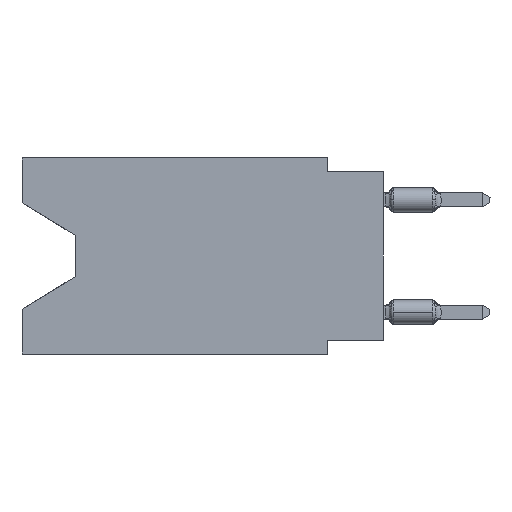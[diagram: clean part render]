
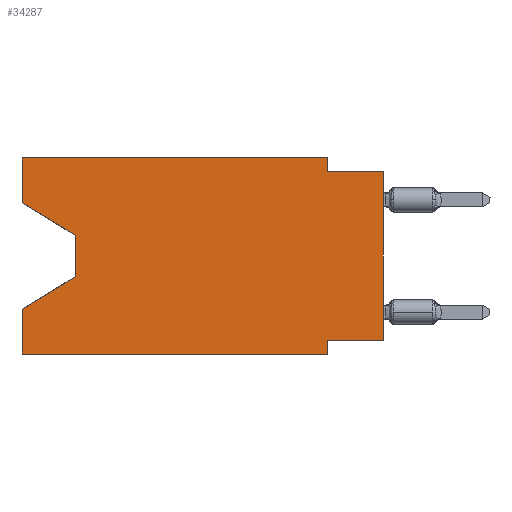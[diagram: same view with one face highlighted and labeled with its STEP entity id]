
A CAD part, left-side view. The second image highlights one B-rep face of the part: STEP entity #34287.
In plain terms, the highlighted planar face has unit normal (-1, 0, 0).
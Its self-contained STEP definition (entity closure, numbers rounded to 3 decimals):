
#469 = ORIENTED_EDGE ( 'NONE', *, *, #32778, .F. ) ;
#590 = FACE_OUTER_BOUND ( 'NONE', #2117, .T. ) ;
#646 = EDGE_CURVE ( 'NONE', #11624, #26078, #7148, .T. ) ;
#716 = ORIENTED_EDGE ( 'NONE', *, *, #38335, .T. ) ;
#778 = VERTEX_POINT ( 'NONE', #39962 ) ;
#858 = ORIENTED_EDGE ( 'NONE', *, *, #14081, .F. ) ;
#910 = CARTESIAN_POINT ( 'NONE',  ( 0., 16.383, 0. ) ) ;
#954 = LINE ( 'NONE', #35859, #6596 ) ;
#1358 = VECTOR ( 'NONE', #21196, 1000. ) ;
#1748 = CARTESIAN_POINT ( 'NONE',  ( 0., 13.97, -5.385 ) ) ;
#1871 = LINE ( 'NONE', #11490, #7334 ) ;
#2117 = EDGE_LOOP ( 'NONE', ( #20671, #716, #14573, #31623, #4939, #858, #12662, #27804, #28840, #469, #36798, #38176 ) ) ;
#2161 = LINE ( 'NONE', #33700, #25986 ) ;
#2420 = LINE ( 'NONE', #15163, #4407 ) ;
#3479 = DIRECTION ( 'NONE',  ( 0., 0., -1. ) ) ;
#3521 = EDGE_CURVE ( 'NONE', #37720, #25284, #1871, .T. ) ;
#4067 = VERTEX_POINT ( 'NONE', #38963 ) ;
#4234 = EDGE_CURVE ( 'NONE', #17017, #778, #39991, .T. ) ;
#4407 = VECTOR ( 'NONE', #27920, 1000. ) ;
#4557 = CARTESIAN_POINT ( 'NONE',  ( 0., 16.383, -8.89 ) ) ;
#4939 = ORIENTED_EDGE ( 'NONE', *, *, #33364, .T. ) ;
#5390 = VECTOR ( 'NONE', #20342, 1000. ) ;
#6102 = CARTESIAN_POINT ( 'NONE',  ( 0., 2.54, 0. ) ) ;
#6384 = VECTOR ( 'NONE', #31040, 1000. ) ;
#6531 = VECTOR ( 'NONE', #20181, 1000. ) ;
#6596 = VECTOR ( 'NONE', #3479, 1000. ) ;
#6736 = DIRECTION ( 'NONE',  ( 0., 0., 1. ) ) ;
#7148 = LINE ( 'NONE', #23651, #18880 ) ;
#7334 = VECTOR ( 'NONE', #12125, 1000. ) ;
#7954 = VECTOR ( 'NONE', #6736, 1000. ) ;
#7988 = CARTESIAN_POINT ( 'NONE',  ( 0., 0., -8.255 ) ) ;
#8026 = CARTESIAN_POINT ( 'NONE',  ( 0., 16.383, 0. ) ) ;
#8684 = CARTESIAN_POINT ( 'NONE',  ( 0., 2.54, 0. ) ) ;
#10314 = CARTESIAN_POINT ( 'NONE',  ( 0., 2.54, -8.255 ) ) ;
#11335 = VERTEX_POINT ( 'NONE', #14252 ) ;
#11345 = EDGE_CURVE ( 'NONE', #4067, #39904, #26813, .T. ) ;
#11490 = CARTESIAN_POINT ( 'NONE',  ( 0., 0., -0.635 ) ) ;
#11589 = CARTESIAN_POINT ( 'NONE',  ( 0., 16.383, 0. ) ) ;
#11623 = LINE ( 'NONE', #30629, #28536 ) ;
#11624 = VERTEX_POINT ( 'NONE', #38499 ) ;
#12125 = DIRECTION ( 'NONE',  ( 0., -1., 0. ) ) ;
#12662 = ORIENTED_EDGE ( 'NONE', *, *, #11345, .F. ) ;
#13435 = DIRECTION ( 'NONE',  ( 0., -0.855, -0.519 ) ) ;
#14081 = EDGE_CURVE ( 'NONE', #39904, #11335, #2161, .T. ) ;
#14186 = EDGE_CURVE ( 'NONE', #4067, #25284, #34133, .T. ) ;
#14252 = CARTESIAN_POINT ( 'NONE',  ( 0., 2.54, -8.89 ) ) ;
#14573 = ORIENTED_EDGE ( 'NONE', *, *, #30015, .T. ) ;
#14727 = LINE ( 'NONE', #11589, #1358 ) ;
#15163 = CARTESIAN_POINT ( 'NONE',  ( 0., 16.383, -8.89 ) ) ;
#17017 = VERTEX_POINT ( 'NONE', #4557 ) ;
#17261 = VERTEX_POINT ( 'NONE', #18448 ) ;
#18448 = CARTESIAN_POINT ( 'NONE',  ( 0., 16.383, 0. ) ) ;
#18880 = VECTOR ( 'NONE', #13435, 1000. ) ;
#19621 = CARTESIAN_POINT ( 'NONE',  ( 0., 16.383, 0. ) ) ;
#20181 = DIRECTION ( 'NONE',  ( 0., 0., 1. ) ) ;
#20342 = DIRECTION ( 'NONE',  ( 0., 0., 1. ) ) ;
#20671 = ORIENTED_EDGE ( 'NONE', *, *, #646, .T. ) ;
#20745 = DIRECTION ( 'NONE',  ( 0., 1., 0. ) ) ;
#21196 = DIRECTION ( 'NONE',  ( 0., -1., 0. ) ) ;
#23651 = CARTESIAN_POINT ( 'NONE',  ( 0., 16.383, -2.038 ) ) ;
#24073 = CARTESIAN_POINT ( 'NONE',  ( 0., 2.54, -0.635 ) ) ;
#24366 = DIRECTION ( 'NONE',  ( 0., 0.855, -0.519 ) ) ;
#25284 = VERTEX_POINT ( 'NONE', #40698 ) ;
#25986 = VECTOR ( 'NONE', #31192, 1000. ) ;
#26078 = VERTEX_POINT ( 'NONE', #29476 ) ;
#26813 = LINE ( 'NONE', #7988, #39894 ) ;
#27233 = CARTESIAN_POINT ( 'NONE',  ( 0., 0., 0. ) ) ;
#27804 = ORIENTED_EDGE ( 'NONE', *, *, #14186, .T. ) ;
#27920 = DIRECTION ( 'NONE',  ( 0., -1., 0. ) ) ;
#28199 = EDGE_CURVE ( 'NONE', #17261, #41174, #14727, .T. ) ;
#28536 = VECTOR ( 'NONE', #24366, 1000. ) ;
#28840 = ORIENTED_EDGE ( 'NONE', *, *, #3521, .F. ) ;
#29476 = CARTESIAN_POINT ( 'NONE',  ( 0., 13.97, -3.505 ) ) ;
#30015 = EDGE_CURVE ( 'NONE', #30370, #778, #11623, .T. ) ;
#30370 = VERTEX_POINT ( 'NONE', #1748 ) ;
#30629 = CARTESIAN_POINT ( 'NONE',  ( 0., 13.97, -5.385 ) ) ;
#30838 = LINE ( 'NONE', #8684, #6384 ) ;
#31040 = DIRECTION ( 'NONE',  ( 0., 0., -1. ) ) ;
#31089 = AXIS2_PLACEMENT_3D ( 'NONE', #19621, #32356, #35503 ) ;
#31192 = DIRECTION ( 'NONE',  ( 0., 0., -1. ) ) ;
#31623 = ORIENTED_EDGE ( 'NONE', *, *, #4234, .F. ) ;
#31734 = PLANE ( 'NONE',  #31089 ) ;
#32356 = DIRECTION ( 'NONE',  ( 1., 0., 0. ) ) ;
#32778 = EDGE_CURVE ( 'NONE', #41174, #37720, #30838, .T. ) ;
#33364 = EDGE_CURVE ( 'NONE', #17017, #11335, #2420, .T. ) ;
#33700 = CARTESIAN_POINT ( 'NONE',  ( 0., 2.54, -8.89 ) ) ;
#34133 = LINE ( 'NONE', #27233, #7954 ) ;
#34287 = ADVANCED_FACE ( 'NONE', ( #590 ), #31734, .F. ) ;
#35503 = DIRECTION ( 'NONE',  ( 0., 0., -1. ) ) ;
#35859 = CARTESIAN_POINT ( 'NONE',  ( 0., 13.97, -3.505 ) ) ;
#36674 = LINE ( 'NONE', #8026, #6531 ) ;
#36798 = ORIENTED_EDGE ( 'NONE', *, *, #28199, .F. ) ;
#37259 = EDGE_CURVE ( 'NONE', #11624, #17261, #36674, .T. ) ;
#37720 = VERTEX_POINT ( 'NONE', #24073 ) ;
#38176 = ORIENTED_EDGE ( 'NONE', *, *, #37259, .F. ) ;
#38335 = EDGE_CURVE ( 'NONE', #26078, #30370, #954, .T. ) ;
#38499 = CARTESIAN_POINT ( 'NONE',  ( 0., 16.383, -2.038 ) ) ;
#38963 = CARTESIAN_POINT ( 'NONE',  ( 0., 0., -8.255 ) ) ;
#39894 = VECTOR ( 'NONE', #20745, 1000. ) ;
#39904 = VERTEX_POINT ( 'NONE', #10314 ) ;
#39962 = CARTESIAN_POINT ( 'NONE',  ( 0., 16.383, -6.852 ) ) ;
#39991 = LINE ( 'NONE', #910, #5390 ) ;
#40698 = CARTESIAN_POINT ( 'NONE',  ( 0., 0., -0.635 ) ) ;
#41174 = VERTEX_POINT ( 'NONE', #6102 ) ;
